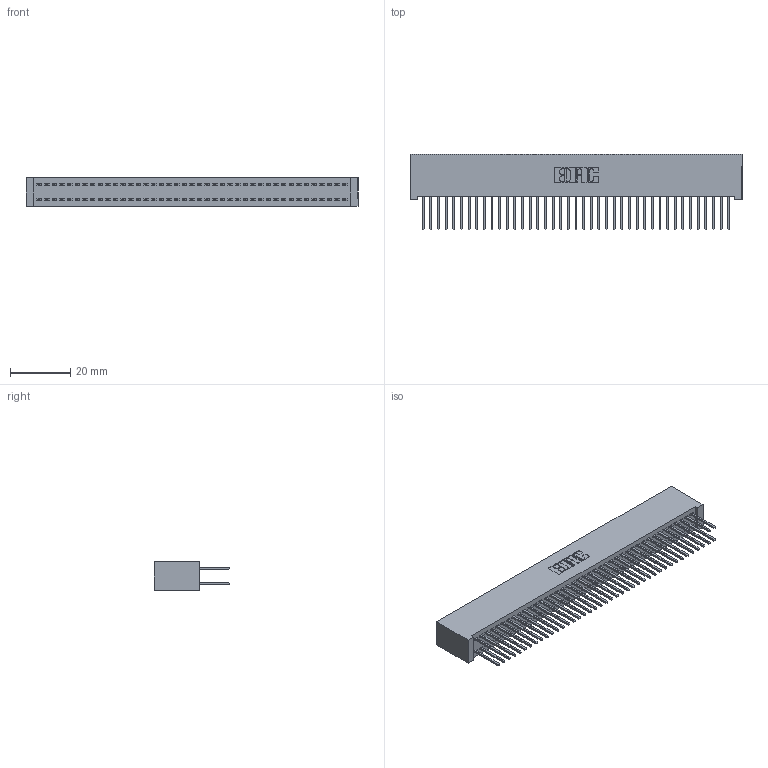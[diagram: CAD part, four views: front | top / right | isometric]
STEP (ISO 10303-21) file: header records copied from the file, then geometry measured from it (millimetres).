
FILE_DESCRIPTION (( 'STEP AP203' ), '1' );
FILE_NAME ('392-082-523-201.STEP', '2018-08-18T03:30:51', ( '' ), ( '' ), 'SwSTEP 2.0', 'SolidWorks 2016', '' );
FILE_SCHEMA (( 'CONFIG_CONTROL_DESIGN' ));
Length unit declared in the file: inch
Products named in the file (3): 342 Part_Lugless; 345-292-001_345-293-123; 392-082-523-201
Assembly tree (83 placements, depth 2):
  392-082-523-201
    342 Part_Lugless
    345-292-001_345-293-123  x82
Bounding box: 110.39 x 25.15 x 9.4 mm (x, y, z)
Volume: 10521.2 mm3; surface area: 18262.5 mm2
Topology: 83 solids, 83 shells, 4366 faces, 12985 edges, 8546 vertices
Faces by surface type: plane 3014, cylinder 1352
Entity records: 26115 total; most frequent: CARTESIAN_POINT 4326, ORIENTED_EDGE 4262, DIRECTION 3691, EDGE_CURVE 2131, VECTOR 2011, LINE 2011, VERTEX_POINT 1418, AXIS2_PLACEMENT_3D 840
